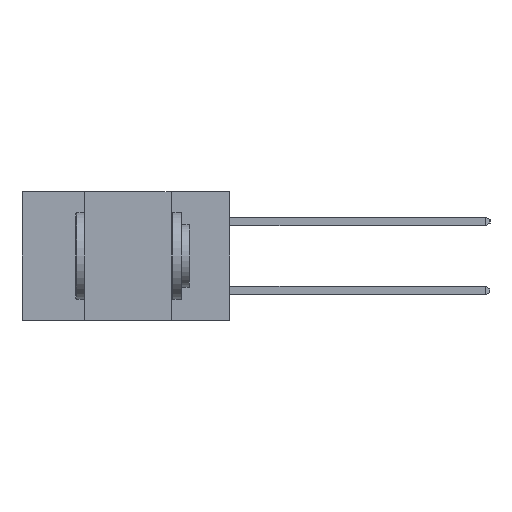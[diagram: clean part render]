
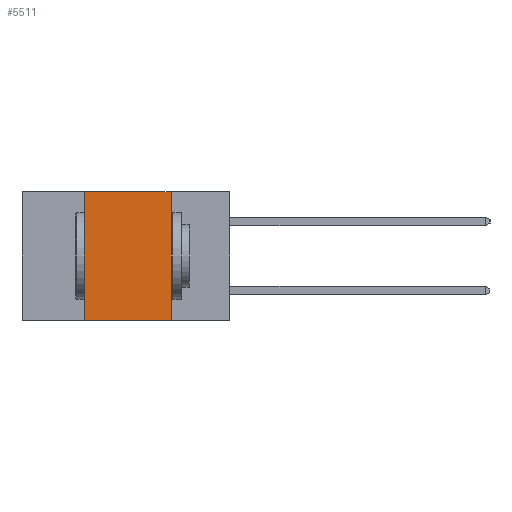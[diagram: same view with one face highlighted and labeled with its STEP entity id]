
A CAD part, left-side view. The second image highlights one B-rep face of the part: STEP entity #5511.
In plain terms, the highlighted planar face has unit normal (-1, 0, 0).
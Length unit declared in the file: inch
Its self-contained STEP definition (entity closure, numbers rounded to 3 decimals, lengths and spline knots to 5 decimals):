
#455 = VECTOR ( 'NONE', #2478, 39.37008 ) ;
#605 = VERTEX_POINT ( 'NONE', #4937 ) ;
#621 = ORIENTED_EDGE ( 'NONE', *, *, #2961, .T. ) ;
#1617 = EDGE_CURVE ( 'NONE', #1681, #6662, #4700, .T. ) ;
#1681 = VERTEX_POINT ( 'NONE', #15657 ) ;
#1930 = CARTESIAN_POINT ( 'NONE',  ( 0., 0.17, -0.37 ) ) ;
#2478 = DIRECTION ( 'NONE',  ( 0., 0., 1. ) ) ;
#2961 = EDGE_CURVE ( 'NONE', #605, #16950, #18508, .T. ) ;
#4700 = LINE ( 'NONE', #16741, #8385 ) ;
#4937 = CARTESIAN_POINT ( 'NONE',  ( 0., 0.42, -0.37 ) ) ;
#4972 = DIRECTION ( 'NONE',  ( 1., 0., 0. ) ) ;
#5263 = LINE ( 'NONE', #10299, #455 ) ;
#5511 = ADVANCED_FACE ( 'NONE', ( #5604 ), #16181, .F. ) ;
#5604 = FACE_OUTER_BOUND ( 'NONE', #14416, .T. ) ;
#6662 = VERTEX_POINT ( 'NONE', #14862 ) ;
#7146 = ORIENTED_EDGE ( 'NONE', *, *, #9664, .F. ) ;
#8105 = ORIENTED_EDGE ( 'NONE', *, *, #1617, .F. ) ;
#8385 = VECTOR ( 'NONE', #9049, 39.37008 ) ;
#9049 = DIRECTION ( 'NONE',  ( 0., -1., 0. ) ) ;
#9664 = EDGE_CURVE ( 'NONE', #6662, #16950, #17812, .T. ) ;
#10048 = VECTOR ( 'NONE', #14162, 39.37008 ) ;
#10299 = CARTESIAN_POINT ( 'NONE',  ( 0., 0.42, 0. ) ) ;
#12214 = ORIENTED_EDGE ( 'NONE', *, *, #18983, .F. ) ;
#13921 = VECTOR ( 'NONE', #17844, 39.37008 ) ;
#14162 = DIRECTION ( 'NONE',  ( 0., 0., -1. ) ) ;
#14416 = EDGE_LOOP ( 'NONE', ( #7146, #8105, #12214, #621 ) ) ;
#14862 = CARTESIAN_POINT ( 'NONE',  ( 0., 0.17, 0. ) ) ;
#15657 = CARTESIAN_POINT ( 'NONE',  ( 0., 0.42, 0. ) ) ;
#16181 = PLANE ( 'NONE',  #19710 ) ;
#16741 = CARTESIAN_POINT ( 'NONE',  ( 0., 0.6, 0. ) ) ;
#16950 = VERTEX_POINT ( 'NONE', #1930 ) ;
#17270 = CARTESIAN_POINT ( 'NONE',  ( 0., 0.17, 0. ) ) ;
#17812 = LINE ( 'NONE', #17270, #10048 ) ;
#17844 = DIRECTION ( 'NONE',  ( 0., -1., 0. ) ) ;
#17912 = CARTESIAN_POINT ( 'NONE',  ( 0., 0.6, -0.37 ) ) ;
#18508 = LINE ( 'NONE', #17912, #13921 ) ;
#18647 = CARTESIAN_POINT ( 'NONE',  ( 0., 0.6, 0. ) ) ;
#18983 = EDGE_CURVE ( 'NONE', #605, #1681, #5263, .T. ) ;
#19710 = AXIS2_PLACEMENT_3D ( 'NONE', #18647, #4972, #20113 ) ;
#20113 = DIRECTION ( 'NONE',  ( 0., 0., -1. ) ) ;
